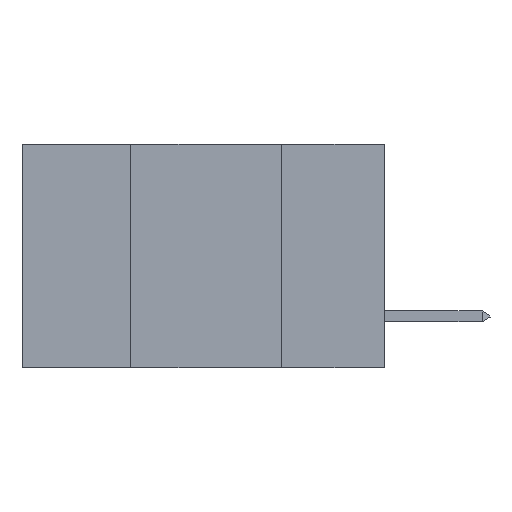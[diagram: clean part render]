
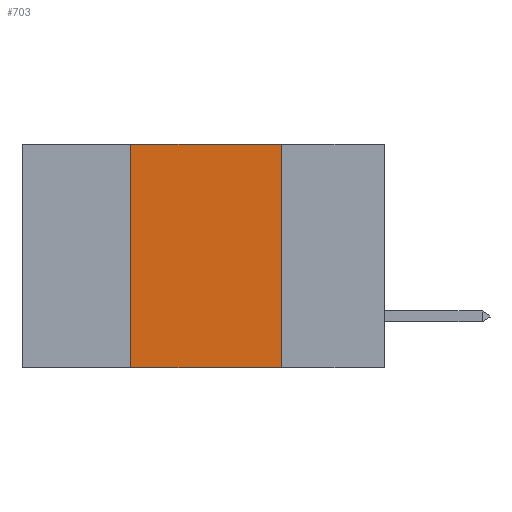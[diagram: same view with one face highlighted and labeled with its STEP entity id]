
A CAD part, left-side view. The second image highlights one B-rep face of the part: STEP entity #703.
In plain terms, the highlighted planar face has unit normal (-1, 0, 0).
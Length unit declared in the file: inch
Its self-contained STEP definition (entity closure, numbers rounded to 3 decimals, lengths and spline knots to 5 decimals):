
#340 = LINE ( 'NONE', #5996, #9434 ) ;
#533 = CARTESIAN_POINT ( 'NONE',  ( 0., 0.42, 0. ) ) ;
#552 = EDGE_CURVE ( 'NONE', #3157, #4205, #340, .T. ) ;
#703 = ADVANCED_FACE ( 'NONE', ( #7822 ), #5099, .F. ) ;
#1193 = ORIENTED_EDGE ( 'NONE', *, *, #8668, .F. ) ;
#1331 = VECTOR ( 'NONE', #5388, 39.37008 ) ;
#2405 = ORIENTED_EDGE ( 'NONE', *, *, #552, .T. ) ;
#3098 = EDGE_CURVE ( 'NONE', #4771, #3263, #9879, .T. ) ;
#3157 = VERTEX_POINT ( 'NONE', #4259 ) ;
#3263 = VERTEX_POINT ( 'NONE', #5995 ) ;
#4205 = VERTEX_POINT ( 'NONE', #8001 ) ;
#4259 = CARTESIAN_POINT ( 'NONE',  ( 0., 0.42, -0.37 ) ) ;
#4264 = DIRECTION ( 'NONE',  ( 0., 0., 1. ) ) ;
#4515 = AXIS2_PLACEMENT_3D ( 'NONE', #8616, #6359, #14150 ) ;
#4771 = VERTEX_POINT ( 'NONE', #533 ) ;
#4879 = CARTESIAN_POINT ( 'NONE',  ( 0., 0.17, 0. ) ) ;
#5099 = PLANE ( 'NONE',  #4515 ) ;
#5388 = DIRECTION ( 'NONE',  ( 0., -1., 0. ) ) ;
#5716 = EDGE_CURVE ( 'NONE', #3263, #4205, #9619, .T. ) ;
#5996 = CARTESIAN_POINT ( 'NONE',  ( 0., 0.6, -0.37 ) ) ;
#5995 = CARTESIAN_POINT ( 'NONE',  ( 0., 0.17, 0. ) ) ;
#6359 = DIRECTION ( 'NONE',  ( 1., 0., 0. ) ) ;
#7822 = FACE_OUTER_BOUND ( 'NONE', #13983, .T. ) ;
#8001 = CARTESIAN_POINT ( 'NONE',  ( 0., 0.17, -0.37 ) ) ;
#8616 = CARTESIAN_POINT ( 'NONE',  ( 0., 0.6, 0. ) ) ;
#8668 = EDGE_CURVE ( 'NONE', #3157, #4771, #11790, .T. ) ;
#8799 = VECTOR ( 'NONE', #4264, 39.37008 ) ;
#9434 = VECTOR ( 'NONE', #9516, 39.37008 ) ;
#9516 = DIRECTION ( 'NONE',  ( 0., -1., 0. ) ) ;
#9619 = LINE ( 'NONE', #4879, #12357 ) ;
#9879 = LINE ( 'NONE', #13459, #1331 ) ;
#11223 = CARTESIAN_POINT ( 'NONE',  ( 0., 0.42, 0. ) ) ;
#11332 = DIRECTION ( 'NONE',  ( 0., 0., -1. ) ) ;
#11790 = LINE ( 'NONE', #11223, #8799 ) ;
#12357 = VECTOR ( 'NONE', #11332, 39.37008 ) ;
#12846 = ORIENTED_EDGE ( 'NONE', *, *, #3098, .F. ) ;
#13076 = ORIENTED_EDGE ( 'NONE', *, *, #5716, .F. ) ;
#13459 = CARTESIAN_POINT ( 'NONE',  ( 0., 0.6, 0. ) ) ;
#13983 = EDGE_LOOP ( 'NONE', ( #13076, #12846, #1193, #2405 ) ) ;
#14150 = DIRECTION ( 'NONE',  ( 0., 0., -1. ) ) ;
